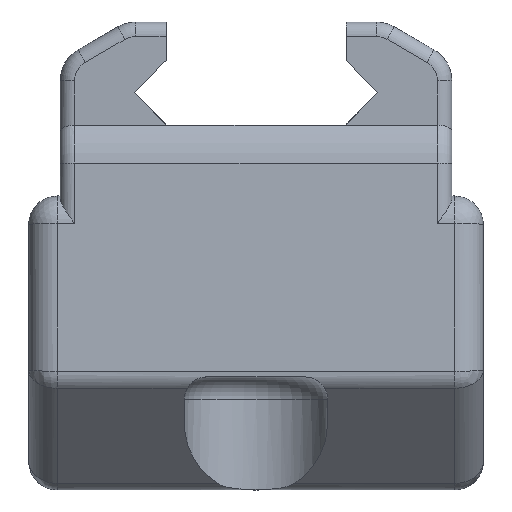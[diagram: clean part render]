
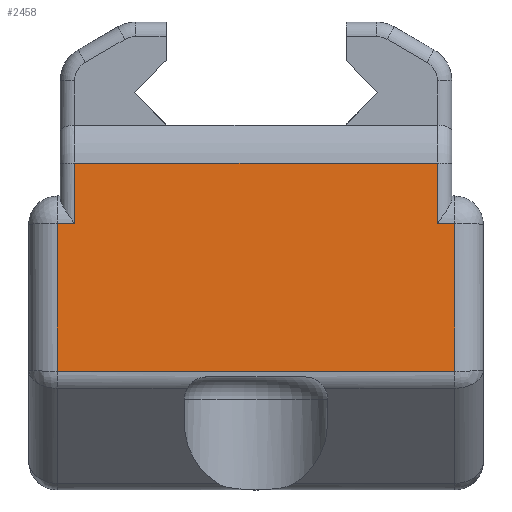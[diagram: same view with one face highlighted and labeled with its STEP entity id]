
A CAD part, front view. The second image highlights one B-rep face of the part: STEP entity #2458.
In plain terms, the highlighted planar face has unit normal (0, -0.999, 0.044).
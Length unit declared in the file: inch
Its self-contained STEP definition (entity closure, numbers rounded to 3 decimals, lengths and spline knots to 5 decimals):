
#90=PLANE('',#2631);
#179=FACE_OUTER_BOUND('',#321,.T.);
#321=EDGE_LOOP('',(#1790,#1791,#1792,#1793,#1794,#1795,#1796,#1797));
#646=LINE('',#12605,#853);
#647=LINE('',#12608,#854);
#651=LINE('',#12619,#858);
#652=LINE('',#12621,#859);
#653=LINE('',#12623,#860);
#654=LINE('',#12625,#861);
#655=LINE('',#12626,#862);
#656=LINE('',#12627,#863);
#853=VECTOR('',#2996,0.3937);
#854=VECTOR('',#2999,0.3937);
#858=VECTOR('',#3007,0.3937);
#859=VECTOR('',#3008,0.3937);
#860=VECTOR('',#3009,0.3937);
#861=VECTOR('',#3010,0.3937);
#862=VECTOR('',#3011,0.3937);
#863=VECTOR('',#3012,0.3937);
#1091=VERTEX_POINT('',#12560);
#1093=VERTEX_POINT('',#12594);
#1094=VERTEX_POINT('',#12607);
#1098=VERTEX_POINT('',#12617);
#1099=VERTEX_POINT('',#12618);
#1100=VERTEX_POINT('',#12620);
#1101=VERTEX_POINT('',#12622);
#1102=VERTEX_POINT('',#12624);
#1349=EDGE_CURVE('',#1093,#1091,#646,.T.);
#1350=EDGE_CURVE('',#1094,#1091,#647,.T.);
#1355=EDGE_CURVE('',#1098,#1099,#651,.T.);
#1356=EDGE_CURVE('',#1100,#1098,#652,.T.);
#1357=EDGE_CURVE('',#1101,#1100,#653,.T.);
#1358=EDGE_CURVE('',#1102,#1101,#654,.T.);
#1359=EDGE_CURVE('',#1094,#1102,#655,.T.);
#1360=EDGE_CURVE('',#1099,#1093,#656,.T.);
#1790=ORIENTED_EDGE('',*,*,#1355,.F.);
#1791=ORIENTED_EDGE('',*,*,#1356,.F.);
#1792=ORIENTED_EDGE('',*,*,#1357,.F.);
#1793=ORIENTED_EDGE('',*,*,#1358,.F.);
#1794=ORIENTED_EDGE('',*,*,#1359,.F.);
#1795=ORIENTED_EDGE('',*,*,#1350,.T.);
#1796=ORIENTED_EDGE('',*,*,#1349,.F.);
#1797=ORIENTED_EDGE('',*,*,#1360,.F.);
#2458=ADVANCED_FACE('',(#179),#90,.T.);
#2631=AXIS2_PLACEMENT_3D('',#12616,#3005,#3006);
#2996=DIRECTION('',(0.,0.044,0.999));
#2999=DIRECTION('',(-1.,0.,0.));
#3005=DIRECTION('center_axis',(0.,-0.999,
0.044));
#3006=DIRECTION('ref_axis',(0.,0.044,0.999));
#3007=DIRECTION('',(0.,0.044,0.999));
#3008=DIRECTION('',(-1.,0.,0.));
#3009=DIRECTION('',(0.,-0.044,-0.999));
#3010=DIRECTION('',(1.,0.,0.));
#3011=DIRECTION('',(0.,-0.044,-0.999));
#3012=DIRECTION('',(1.,0.,0.));
#12560=CARTESIAN_POINT('',(-0.64655,-0.74752,0.75979));
#12594=CARTESIAN_POINT('',(-0.64655,-0.75689,0.54948));
#12605=CARTESIAN_POINT('',(-0.64655,-0.56772,4.79702));
#12607=CARTESIAN_POINT('',(0.6172,-0.74752,0.75979));
#12608=CARTESIAN_POINT('',(0.32618,-0.74752,0.75979));
#12616=CARTESIAN_POINT('Origin',(-0.01484,-0.39823,
8.60287));
#12617=CARTESIAN_POINT('',(-0.70617,-0.7798,0.03487));
#12618=CARTESIAN_POINT('',(-0.70617,-0.75689,0.54948));
#12619=CARTESIAN_POINT('',(-0.70617,-0.60876,3.87558));
#12620=CARTESIAN_POINT('',(0.6765,-0.7798,0.03487));
#12621=CARTESIAN_POINT('',(-0.24318,-0.7798,0.03487));
#12622=CARTESIAN_POINT('',(0.6765,-0.75689,0.54948));
#12623=CARTESIAN_POINT('',(0.6765,-0.57354,4.66634));
#12624=CARTESIAN_POINT('',(0.6172,-0.75689,0.54948));
#12625=CARTESIAN_POINT('',(-0.11917,-0.75689,0.54948));
#12626=CARTESIAN_POINT('',(0.6172,-0.56772,4.79702));
#12627=CARTESIAN_POINT('',(-0.11917,-0.75689,0.54948));
